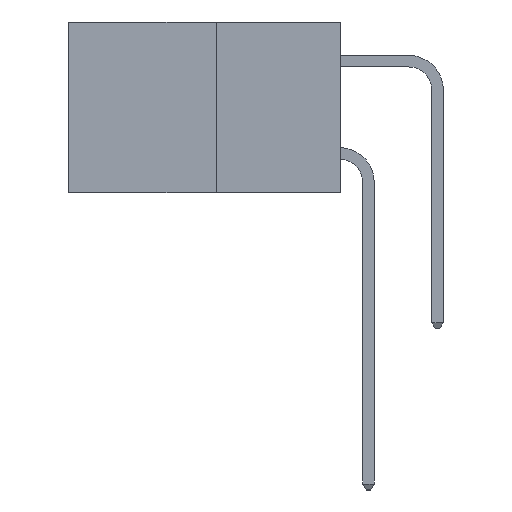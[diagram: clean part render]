
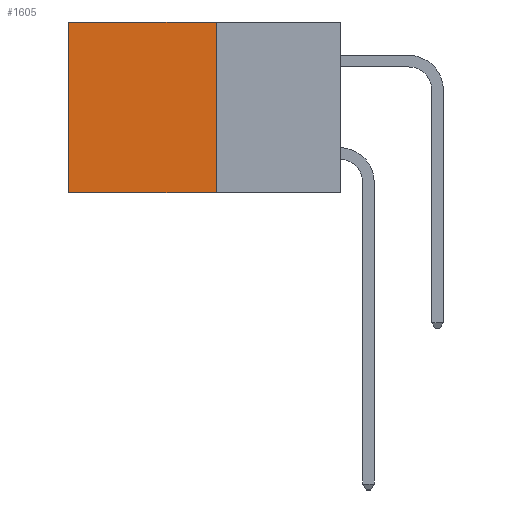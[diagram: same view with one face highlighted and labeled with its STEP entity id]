
A CAD part, left-side view. The second image highlights one B-rep face of the part: STEP entity #1605.
In plain terms, the highlighted planar face has unit normal (-1, 0, 0).
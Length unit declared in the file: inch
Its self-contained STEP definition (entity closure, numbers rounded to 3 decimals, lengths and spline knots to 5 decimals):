
#493 = EDGE_CURVE ( 'NONE', #2593, #19324, #3155, .T. ) ;
#1605 = ADVANCED_FACE ( 'NONE', ( #15478 ), #16589, .F. ) ;
#2593 = VERTEX_POINT ( 'NONE', #28345 ) ;
#3155 = LINE ( 'NONE', #16514, #15926 ) ;
#3461 = ORIENTED_EDGE ( 'NONE', *, *, #30876, .T. ) ;
#4215 = EDGE_CURVE ( 'NONE', #18867, #15234, #28060, .T. ) ;
#4827 = DIRECTION ( 'NONE',  ( 0., 0., -1. ) ) ;
#6755 = CARTESIAN_POINT ( 'NONE',  ( 0.277, 0.27, -0.37 ) ) ;
#8759 = AXIS2_PLACEMENT_3D ( 'NONE', #16614, #16505, #16447 ) ;
#8774 = CARTESIAN_POINT ( 'NONE',  ( 0.277, 0.27, -0.37 ) ) ;
#9327 = CARTESIAN_POINT ( 'NONE',  ( 0.277, 0.27, -0.37 ) ) ;
#9775 = CARTESIAN_POINT ( 'NONE',  ( 0.277, 0.59, 0. ) ) ;
#11596 = DIRECTION ( 'NONE',  ( 0., 0., -1. ) ) ;
#11738 = EDGE_CURVE ( 'NONE', #2593, #18867, #29249, .T. ) ;
#15234 = VERTEX_POINT ( 'NONE', #19280 ) ;
#15382 = VECTOR ( 'NONE', #23646, 39.37008 ) ;
#15478 = FACE_OUTER_BOUND ( 'NONE', #20503, .T. ) ;
#15926 = VECTOR ( 'NONE', #21298, 39.37008 ) ;
#16447 = DIRECTION ( 'NONE',  ( 0., 0., -1. ) ) ;
#16505 = DIRECTION ( 'NONE',  ( 1., 0., 0. ) ) ;
#16514 = CARTESIAN_POINT ( 'NONE',  ( 0.277, 0.27, 0. ) ) ;
#16589 = PLANE ( 'NONE',  #8759 ) ;
#16614 = CARTESIAN_POINT ( 'NONE',  ( 0.277, 0.27, -0.37 ) ) ;
#18867 = VERTEX_POINT ( 'NONE', #8774 ) ;
#19161 = VECTOR ( 'NONE', #4827, 39.37008 ) ;
#19174 = CARTESIAN_POINT ( 'NONE',  ( 0.277, 0.59, -0.37 ) ) ;
#19280 = CARTESIAN_POINT ( 'NONE',  ( 0.277, 0.59, -0.37 ) ) ;
#19324 = VERTEX_POINT ( 'NONE', #9775 ) ;
#20503 = EDGE_LOOP ( 'NONE', ( #3461, #27150, #24911, #21386 ) ) ;
#21298 = DIRECTION ( 'NONE',  ( 0., 1., 0. ) ) ;
#21386 = ORIENTED_EDGE ( 'NONE', *, *, #493, .T. ) ;
#22937 = VECTOR ( 'NONE', #11596, 39.37008 ) ;
#23646 = DIRECTION ( 'NONE',  ( 0., 1., 0. ) ) ;
#24911 = ORIENTED_EDGE ( 'NONE', *, *, #11738, .F. ) ;
#26237 = LINE ( 'NONE', #19174, #19161 ) ;
#27150 = ORIENTED_EDGE ( 'NONE', *, *, #4215, .F. ) ;
#28060 = LINE ( 'NONE', #9327, #15382 ) ;
#28345 = CARTESIAN_POINT ( 'NONE',  ( 0.277, 0.27, 0. ) ) ;
#29249 = LINE ( 'NONE', #6755, #22937 ) ;
#30876 = EDGE_CURVE ( 'NONE', #19324, #15234, #26237, .T. ) ;
